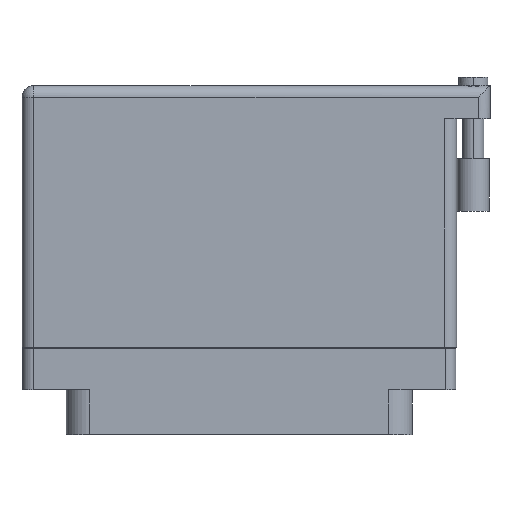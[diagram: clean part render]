
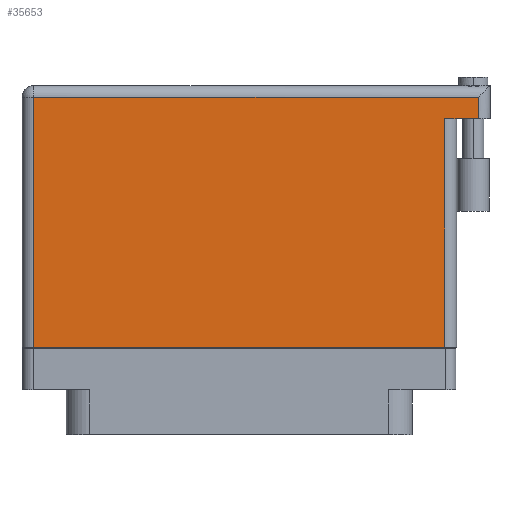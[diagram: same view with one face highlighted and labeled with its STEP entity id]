
A CAD part, front view. The second image highlights one B-rep face of the part: STEP entity #35653.
In plain terms, the highlighted face is planar.
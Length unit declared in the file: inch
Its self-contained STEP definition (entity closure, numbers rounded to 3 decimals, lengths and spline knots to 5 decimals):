
#274 = DIRECTION ( 'NONE',  ( 0., -1., 0. ) ) ;
#916 = VERTEX_POINT ( 'NONE', #27392 ) ;
#1300 = EDGE_LOOP ( 'NONE', ( #17726, #33829, #39592, #32826, #26940, #23112 ) ) ;
#7402 = CARTESIAN_POINT ( 'NONE',  ( 1.43, 1.396, 0.4495 ) ) ;
#7983 = VECTOR ( 'NONE', #30051, 39.37008 ) ;
#9055 = VERTEX_POINT ( 'NONE', #42913 ) ;
#9265 = EDGE_CURVE ( 'NONE', #41322, #47057, #30913, .T. ) ;
#10070 = VERTEX_POINT ( 'NONE', #7402 ) ;
#10214 = EDGE_CURVE ( 'NONE', #47057, #47421, #36791, .T. ) ;
#10542 = DIRECTION ( 'NONE',  ( -1., 0., 0. ) ) ;
#10602 = DIRECTION ( 'NONE',  ( 0., 1., 0. ) ) ;
#11743 = CARTESIAN_POINT ( 'NONE',  ( -1.3, 1.466, 0.4495 ) ) ;
#13010 = DIRECTION ( 'NONE',  ( 1., 0., 0. ) ) ;
#13154 = EDGE_CURVE ( 'NONE', #916, #10070, #35997, .T. ) ;
#13672 = LINE ( 'NONE', #32053, #41170 ) ;
#15192 = FACE_OUTER_BOUND ( 'NONE', #1300, .T. ) ;
#16682 = VECTOR ( 'NONE', #13010, 39.37008 ) ;
#17726 = ORIENTED_EDGE ( 'NONE', *, *, #10214, .T. ) ;
#20520 = CARTESIAN_POINT ( 'NONE',  ( -1.3, -0.1, 0.4495 ) ) ;
#22347 = EDGE_CURVE ( 'NONE', #916, #9055, #46768, .T. ) ;
#23112 = ORIENTED_EDGE ( 'NONE', *, *, #9265, .T. ) ;
#25865 = DIRECTION ( 'NONE',  ( 0., 0., -1. ) ) ;
#26811 = EDGE_CURVE ( 'NONE', #47421, #9055, #29161, .T. ) ;
#26940 = ORIENTED_EDGE ( 'NONE', *, *, #32163, .T. ) ;
#27170 = DIRECTION ( 'NONE',  ( -1., 0., 0. ) ) ;
#27392 = CARTESIAN_POINT ( 'NONE',  ( 1.43, 1.269, 0.4495 ) ) ;
#28550 = CARTESIAN_POINT ( 'NONE',  ( 1.43, 1.466, 0.4495 ) ) ;
#29161 = LINE ( 'NONE', #44319, #7983 ) ;
#30051 = DIRECTION ( 'NONE',  ( 0., 1., 0. ) ) ;
#30913 = LINE ( 'NONE', #40194, #36047 ) ;
#31027 = CARTESIAN_POINT ( 'NONE',  ( 1.5, 1.269, 0.4495 ) ) ;
#31805 = CARTESIAN_POINT ( 'NONE',  ( -1.23, -0.1, 0.4495 ) ) ;
#32053 = CARTESIAN_POINT ( 'NONE',  ( -1.3, 1.396, 0.4495 ) ) ;
#32163 = EDGE_CURVE ( 'NONE', #10070, #41322, #13672, .T. ) ;
#32826 = ORIENTED_EDGE ( 'NONE', *, *, #13154, .T. ) ;
#33829 = ORIENTED_EDGE ( 'NONE', *, *, #26811, .T. ) ;
#33907 = PLANE ( 'NONE',  #44948 ) ;
#34899 = VECTOR ( 'NONE', #10602, 39.37008 ) ;
#35653 = ADVANCED_FACE ( 'NONE', ( #15192 ), #33907, .F. ) ;
#35862 = VECTOR ( 'NONE', #27170, 39.37008 ) ;
#35915 = CARTESIAN_POINT ( 'NONE',  ( -1.23, 1.396, 0.4495 ) ) ;
#35997 = LINE ( 'NONE', #28550, #34899 ) ;
#36047 = VECTOR ( 'NONE', #274, 39.37008 ) ;
#36791 = LINE ( 'NONE', #20520, #16682 ) ;
#39592 = ORIENTED_EDGE ( 'NONE', *, *, #22347, .F. ) ;
#40194 = CARTESIAN_POINT ( 'NONE',  ( -1.23, -0.1, 0.4495 ) ) ;
#41170 = VECTOR ( 'NONE', #10542, 39.37008 ) ;
#41322 = VERTEX_POINT ( 'NONE', #35915 ) ;
#42913 = CARTESIAN_POINT ( 'NONE',  ( 1.23, 1.269, 0.4495 ) ) ;
#44319 = CARTESIAN_POINT ( 'NONE',  ( 1.23, 1.269, 0.4495 ) ) ;
#44606 = DIRECTION ( 'NONE',  ( -1., 0., 0. ) ) ;
#44948 = AXIS2_PLACEMENT_3D ( 'NONE', #11743, #25865, #44606 ) ;
#46768 = LINE ( 'NONE', #31027, #35862 ) ;
#47057 = VERTEX_POINT ( 'NONE', #31805 ) ;
#47358 = CARTESIAN_POINT ( 'NONE',  ( 1.23, -0.1, 0.4495 ) ) ;
#47421 = VERTEX_POINT ( 'NONE', #47358 ) ;
